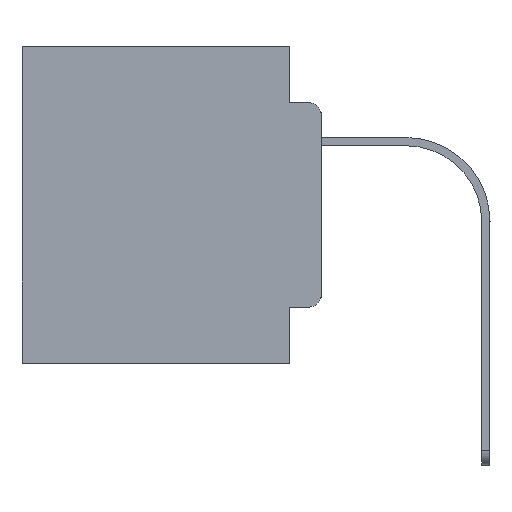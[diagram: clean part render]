
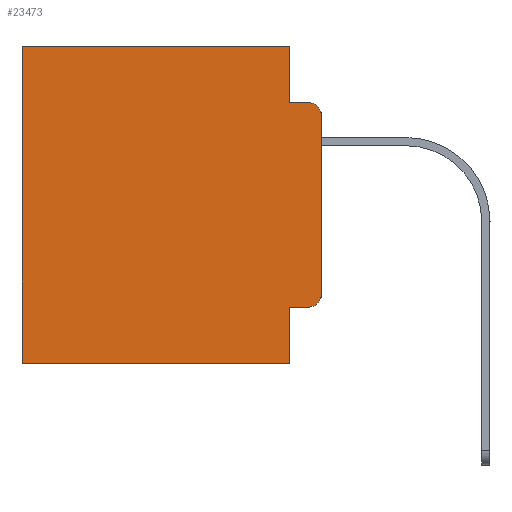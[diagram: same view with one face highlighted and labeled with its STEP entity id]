
A CAD part, left-side view. The second image highlights one B-rep face of the part: STEP entity #23473.
In plain terms, the highlighted planar face has unit normal (-1, 0, 0).
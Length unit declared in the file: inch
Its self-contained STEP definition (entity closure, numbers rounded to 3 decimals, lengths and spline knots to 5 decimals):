
#169 = DIRECTION ( 'NONE',  ( -1., 0., 0. ) ) ;
#430 = CARTESIAN_POINT ( 'NONE',  ( 0.298, 0.051, -0.4115 ) ) ;
#493 = VECTOR ( 'NONE', #11510, 39.37008 ) ;
#932 = ORIENTED_EDGE ( 'NONE', *, *, #6380, .T. ) ;
#1335 = VERTEX_POINT ( 'NONE', #2730 ) ;
#1594 = CARTESIAN_POINT ( 'NONE',  ( 0.298, 0., -0.5 ) ) ;
#1624 = CIRCLE ( 'NONE', #26754, 0.02 ) ;
#1730 = DIRECTION ( 'NONE',  ( 0., 1., 0. ) ) ;
#2119 = EDGE_CURVE ( 'NONE', #17749, #2195, #6054, .T. ) ;
#2120 = CARTESIAN_POINT ( 'NONE',  ( 0.298, 0., -0.3915 ) ) ;
#2195 = VERTEX_POINT ( 'NONE', #2120 ) ;
#2222 = LINE ( 'NONE', #25845, #17729 ) ;
#2715 = VECTOR ( 'NONE', #11183, 39.37008 ) ;
#2730 = CARTESIAN_POINT ( 'NONE',  ( 0.298, 0., -0.1085 ) ) ;
#3468 = CARTESIAN_POINT ( 'NONE',  ( 0.298, 0.473, -0.5 ) ) ;
#3986 = EDGE_CURVE ( 'NONE', #1335, #2195, #27220, .T. ) ;
#5387 = AXIS2_PLACEMENT_3D ( 'NONE', #7096, #24929, #25053 ) ;
#5706 = CARTESIAN_POINT ( 'NONE',  ( 0.298, 0., 0. ) ) ;
#6054 = CIRCLE ( 'NONE', #16821, 0.02 ) ;
#6380 = EDGE_CURVE ( 'NONE', #21575, #11044, #21248, .T. ) ;
#6731 = CARTESIAN_POINT ( 'NONE',  ( 0.298, 0.051, 0. ) ) ;
#6762 = VECTOR ( 'NONE', #15314, 39.37008 ) ;
#6837 = FACE_OUTER_BOUND ( 'NONE', #15917, .T. ) ;
#7057 = VERTEX_POINT ( 'NONE', #3468 ) ;
#7096 = CARTESIAN_POINT ( 'NONE',  ( 0.298, 0., 0. ) ) ;
#7466 = ORIENTED_EDGE ( 'NONE', *, *, #3986, .F. ) ;
#8978 = CARTESIAN_POINT ( 'NONE',  ( 0.298, 0.051, -0.0885 ) ) ;
#9365 = VERTEX_POINT ( 'NONE', #22774 ) ;
#10137 = DIRECTION ( 'NONE',  ( 0., 1., 0. ) ) ;
#11029 = VECTOR ( 'NONE', #14274, 39.37008 ) ;
#11044 = VERTEX_POINT ( 'NONE', #21315 ) ;
#11183 = DIRECTION ( 'NONE',  ( 0., -1., 0. ) ) ;
#11184 = CARTESIAN_POINT ( 'NONE',  ( 0.298, 0.473, 0. ) ) ;
#11242 = EDGE_CURVE ( 'NONE', #24108, #17749, #15679, .T. ) ;
#11388 = ORIENTED_EDGE ( 'NONE', *, *, #23344, .T. ) ;
#11510 = DIRECTION ( 'NONE',  ( 0., -1., 0. ) ) ;
#11575 = CARTESIAN_POINT ( 'NONE',  ( 0.298, 0.02, -0.1085 ) ) ;
#11970 = EDGE_CURVE ( 'NONE', #21575, #9365, #25995, .T. ) ;
#12388 = LINE ( 'NONE', #1594, #19267 ) ;
#12490 = ORIENTED_EDGE ( 'NONE', *, *, #20587, .T. ) ;
#12793 = DIRECTION ( 'NONE',  ( 0., 0., -1. ) ) ;
#12909 = ORIENTED_EDGE ( 'NONE', *, *, #11242, .T. ) ;
#13053 = ORIENTED_EDGE ( 'NONE', *, *, #2119, .T. ) ;
#14002 = CARTESIAN_POINT ( 'NONE',  ( 0.298, 0.051, 0. ) ) ;
#14274 = DIRECTION ( 'NONE',  ( 0., 0., -1. ) ) ;
#14659 = ORIENTED_EDGE ( 'NONE', *, *, #11970, .F. ) ;
#15314 = DIRECTION ( 'NONE',  ( 0., 0., -1. ) ) ;
#15612 = CARTESIAN_POINT ( 'NONE',  ( 0.298, 0.02, -0.0885 ) ) ;
#15679 = LINE ( 'NONE', #20173, #2715 ) ;
#15917 = EDGE_LOOP ( 'NONE', ( #7466, #12490, #19996, #14659, #932, #11388, #21900, #26421, #12909, #13053 ) ) ;
#15921 = VERTEX_POINT ( 'NONE', #21767 ) ;
#16799 = VERTEX_POINT ( 'NONE', #15612 ) ;
#16821 = AXIS2_PLACEMENT_3D ( 'NONE', #16984, #169, #12793 ) ;
#16984 = CARTESIAN_POINT ( 'NONE',  ( 0.298, 0.02, -0.3915 ) ) ;
#17166 = CARTESIAN_POINT ( 'NONE',  ( 0.298, 0., 0. ) ) ;
#17560 = LINE ( 'NONE', #8978, #493 ) ;
#17729 = VECTOR ( 'NONE', #19641, 39.37008 ) ;
#17749 = VERTEX_POINT ( 'NONE', #24262 ) ;
#19267 = VECTOR ( 'NONE', #10137, 39.37008 ) ;
#19500 = LINE ( 'NONE', #11184, #27383 ) ;
#19641 = DIRECTION ( 'NONE',  ( 0., 0., -1. ) ) ;
#19996 = ORIENTED_EDGE ( 'NONE', *, *, #25374, .F. ) ;
#20038 = EDGE_CURVE ( 'NONE', #24108, #15921, #2222, .T. ) ;
#20173 = CARTESIAN_POINT ( 'NONE',  ( 0.298, 0.051, -0.4115 ) ) ;
#20587 = EDGE_CURVE ( 'NONE', #1335, #16799, #1624, .T. ) ;
#21248 = LINE ( 'NONE', #17166, #22865 ) ;
#21315 = CARTESIAN_POINT ( 'NONE',  ( 0.298, 0.473, 0. ) ) ;
#21575 = VERTEX_POINT ( 'NONE', #14002 ) ;
#21767 = CARTESIAN_POINT ( 'NONE',  ( 0.298, 0.051, -0.5 ) ) ;
#21900 = ORIENTED_EDGE ( 'NONE', *, *, #27630, .F. ) ;
#22005 = DIRECTION ( 'NONE',  ( 0., 0., -1. ) ) ;
#22541 = DIRECTION ( 'NONE',  ( 0., 0., -1. ) ) ;
#22774 = CARTESIAN_POINT ( 'NONE',  ( 0.298, 0.051, -0.0885 ) ) ;
#22865 = VECTOR ( 'NONE', #1730, 39.37008 ) ;
#23344 = EDGE_CURVE ( 'NONE', #11044, #7057, #19500, .T. ) ;
#23473 = ADVANCED_FACE ( 'NONE', ( #6837 ), #25199, .F. ) ;
#24108 = VERTEX_POINT ( 'NONE', #430 ) ;
#24262 = CARTESIAN_POINT ( 'NONE',  ( 0.298, 0.02, -0.4115 ) ) ;
#24929 = DIRECTION ( 'NONE',  ( 1., 0., 0. ) ) ;
#25053 = DIRECTION ( 'NONE',  ( 0., 0., -1. ) ) ;
#25199 = PLANE ( 'NONE',  #5387 ) ;
#25374 = EDGE_CURVE ( 'NONE', #9365, #16799, #17560, .T. ) ;
#25845 = CARTESIAN_POINT ( 'NONE',  ( 0.298, 0.051, 0. ) ) ;
#25995 = LINE ( 'NONE', #6731, #6762 ) ;
#26421 = ORIENTED_EDGE ( 'NONE', *, *, #20038, .F. ) ;
#26754 = AXIS2_PLACEMENT_3D ( 'NONE', #11575, #26900, #22541 ) ;
#26900 = DIRECTION ( 'NONE',  ( -1., 0., 0. ) ) ;
#27220 = LINE ( 'NONE', #5706, #11029 ) ;
#27383 = VECTOR ( 'NONE', #22005, 39.37008 ) ;
#27630 = EDGE_CURVE ( 'NONE', #15921, #7057, #12388, .T. ) ;
